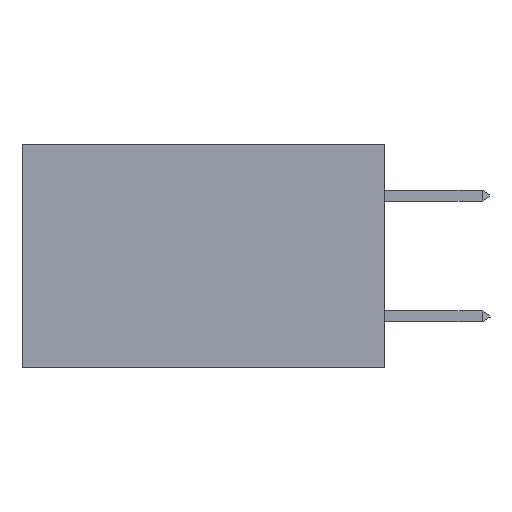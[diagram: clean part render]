
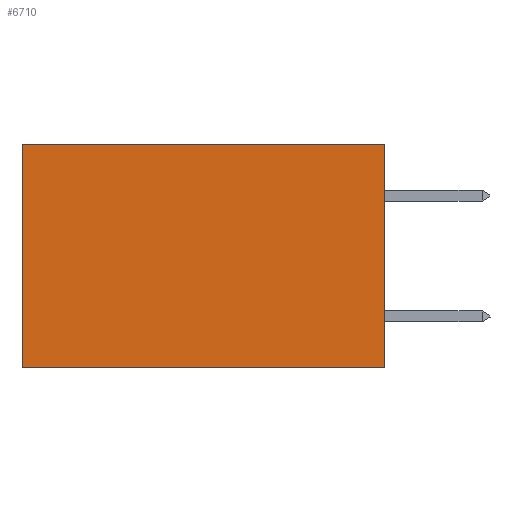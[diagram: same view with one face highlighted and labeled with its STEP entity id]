
A CAD part, left-side view. The second image highlights one B-rep face of the part: STEP entity #6710.
In plain terms, the highlighted planar face has unit normal (-1, 0, 0).
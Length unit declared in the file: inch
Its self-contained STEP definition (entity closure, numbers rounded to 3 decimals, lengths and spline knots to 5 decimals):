
#1089 = CARTESIAN_POINT ( 'NONE',  ( 0.2875, 0., -0.37 ) ) ;
#1581 = EDGE_CURVE ( 'NONE', #27310, #24238, #25178, .T. ) ;
#2138 = VECTOR ( 'NONE', #7700, 39.37008 ) ;
#2429 = CARTESIAN_POINT ( 'NONE',  ( 0.2875, 0.6, 0. ) ) ;
#2441 = DIRECTION ( 'NONE',  ( 0., 0., -1. ) ) ;
#3045 = DIRECTION ( 'NONE',  ( 1., 0., 0. ) ) ;
#4357 = CARTESIAN_POINT ( 'NONE',  ( 0.2875, 0., 0. ) ) ;
#4440 = ORIENTED_EDGE ( 'NONE', *, *, #1581, .F. ) ;
#4679 = VERTEX_POINT ( 'NONE', #13597 ) ;
#5691 = VECTOR ( 'NONE', #16344, 39.37008 ) ;
#6710 = ADVANCED_FACE ( 'NONE', ( #23815 ), #15744, .F. ) ;
#7337 = EDGE_LOOP ( 'NONE', ( #27077, #4440, #9914, #17120 ) ) ;
#7700 = DIRECTION ( 'NONE',  ( 0., 1., 0. ) ) ;
#7982 = VECTOR ( 'NONE', #16040, 39.37008 ) ;
#9914 = ORIENTED_EDGE ( 'NONE', *, *, #27553, .F. ) ;
#12337 = CARTESIAN_POINT ( 'NONE',  ( 0.2875, 0., 0. ) ) ;
#13597 = CARTESIAN_POINT ( 'NONE',  ( 0.2875, 0., 0. ) ) ;
#13654 = CARTESIAN_POINT ( 'NONE',  ( 0.2875, 0., 0. ) ) ;
#13770 = CARTESIAN_POINT ( 'NONE',  ( 0.2875, 0.6, 0. ) ) ;
#15744 = PLANE ( 'NONE',  #15762 ) ;
#15762 = AXIS2_PLACEMENT_3D ( 'NONE', #13654, #3045, #18220 ) ;
#16038 = LINE ( 'NONE', #12337, #2138 ) ;
#16040 = DIRECTION ( 'NONE',  ( 0., 0., -1. ) ) ;
#16344 = DIRECTION ( 'NONE',  ( 0., 1., 0. ) ) ;
#16709 = LINE ( 'NONE', #4357, #27738 ) ;
#17120 = ORIENTED_EDGE ( 'NONE', *, *, #27256, .T. ) ;
#17885 = VERTEX_POINT ( 'NONE', #2429 ) ;
#18220 = DIRECTION ( 'NONE',  ( 0., 0., -1. ) ) ;
#21928 = EDGE_CURVE ( 'NONE', #17885, #24238, #22311, .T. ) ;
#22311 = LINE ( 'NONE', #13770, #7982 ) ;
#23156 = CARTESIAN_POINT ( 'NONE',  ( 0.2875, 0., -0.37 ) ) ;
#23815 = FACE_OUTER_BOUND ( 'NONE', #7337, .T. ) ;
#24238 = VERTEX_POINT ( 'NONE', #27797 ) ;
#25178 = LINE ( 'NONE', #1089, #5691 ) ;
#27077 = ORIENTED_EDGE ( 'NONE', *, *, #21928, .T. ) ;
#27256 = EDGE_CURVE ( 'NONE', #4679, #17885, #16038, .T. ) ;
#27310 = VERTEX_POINT ( 'NONE', #23156 ) ;
#27553 = EDGE_CURVE ( 'NONE', #4679, #27310, #16709, .T. ) ;
#27738 = VECTOR ( 'NONE', #2441, 39.37008 ) ;
#27797 = CARTESIAN_POINT ( 'NONE',  ( 0.2875, 0.6, -0.37 ) ) ;
